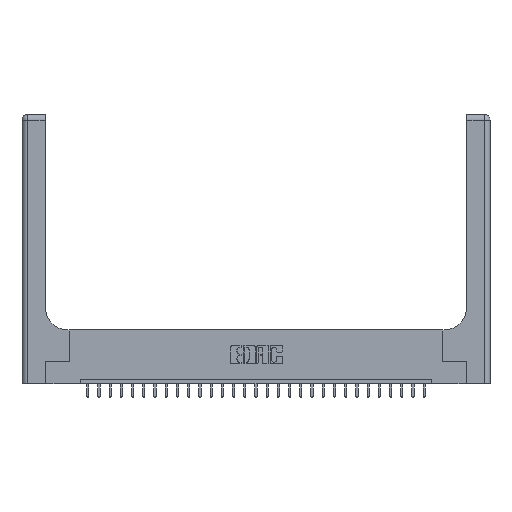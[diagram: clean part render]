
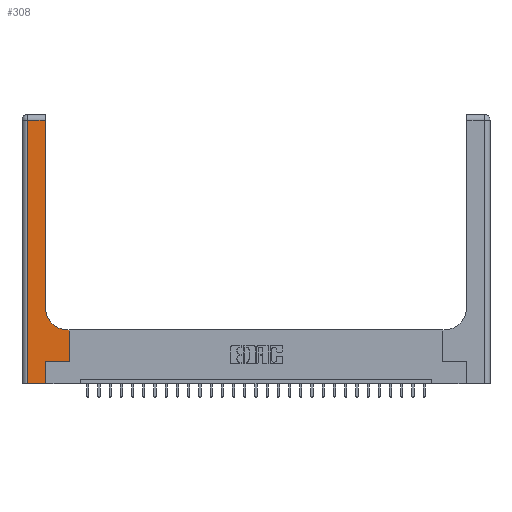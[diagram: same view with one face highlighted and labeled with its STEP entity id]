
A CAD part, top view. The second image highlights one B-rep face of the part: STEP entity #308.
In plain terms, the highlighted planar face has unit normal (0, 0, 1).
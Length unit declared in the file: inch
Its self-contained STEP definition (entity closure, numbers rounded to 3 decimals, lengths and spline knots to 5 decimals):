
#308 = ADVANCED_FACE ( 'NONE', ( #25805 ), #19382, .F. ) ;
#476 = AXIS2_PLACEMENT_3D ( 'NONE', #25495, #11494, #21479 ) ;
#807 = CARTESIAN_POINT ( 'NONE',  ( 0.26, 2.94, 0.37 ) ) ;
#1429 = EDGE_CURVE ( 'NONE', #10382, #23302, #22549, .T. ) ;
#1506 = EDGE_LOOP ( 'NONE', ( #4015, #25766, #17040, #3214, #15412, #5673, #3122, #5263, #17980 ) ) ;
#1592 = VERTEX_POINT ( 'NONE', #12951 ) ;
#2658 = CARTESIAN_POINT ( 'NONE',  ( 0.51, 0.85, 0.37 ) ) ;
#2909 = VECTOR ( 'NONE', #16602, 39.37008 ) ;
#3122 = ORIENTED_EDGE ( 'NONE', *, *, #21930, .T. ) ;
#3214 = ORIENTED_EDGE ( 'NONE', *, *, #24684, .T. ) ;
#3819 = VECTOR ( 'NONE', #23359, 39.37008 ) ;
#3946 = VERTEX_POINT ( 'NONE', #9757 ) ;
#4015 = ORIENTED_EDGE ( 'NONE', *, *, #12102, .T. ) ;
#4040 = CARTESIAN_POINT ( 'NONE',  ( 0.06, 2.94, 0.37 ) ) ;
#4231 = CARTESIAN_POINT ( 'NONE',  ( 0.06, 3., 0.37 ) ) ;
#4755 = CARTESIAN_POINT ( 'NONE',  ( 0.265, 0.25, 0.37 ) ) ;
#5224 = LINE ( 'NONE', #10965, #16913 ) ;
#5263 = ORIENTED_EDGE ( 'NONE', *, *, #16327, .T. ) ;
#5461 = CARTESIAN_POINT ( 'NONE',  ( 0.26, 0.85, 0.37 ) ) ;
#5673 = ORIENTED_EDGE ( 'NONE', *, *, #1429, .T. ) ;
#6763 = CARTESIAN_POINT ( 'NONE',  ( 0.06, 0., 0.37 ) ) ;
#8333 = AXIS2_PLACEMENT_3D ( 'NONE', #2658, #8443, #16576 ) ;
#8377 = LINE ( 'NONE', #18125, #14076 ) ;
#8443 = DIRECTION ( 'NONE',  ( 0., 0., -1. ) ) ;
#9757 = CARTESIAN_POINT ( 'NONE',  ( 0.528, 0.6, 0.37 ) ) ;
#9842 = EDGE_CURVE ( 'NONE', #1592, #21250, #22791, .T. ) ;
#9850 = DIRECTION ( 'NONE',  ( 0., 1., 0. ) ) ;
#9878 = CARTESIAN_POINT ( 'NONE',  ( 0., 2.94, 0.37 ) ) ;
#10382 = VERTEX_POINT ( 'NONE', #21313 ) ;
#10936 = VERTEX_POINT ( 'NONE', #6763 ) ;
#10965 = CARTESIAN_POINT ( 'NONE',  ( 0.265, 0., 0.37 ) ) ;
#11494 = DIRECTION ( 'NONE',  ( 0., 0., -1. ) ) ;
#11501 = VECTOR ( 'NONE', #22801, 39.37008 ) ;
#11527 = EDGE_CURVE ( 'NONE', #16818, #12483, #19607, .T. ) ;
#12102 = EDGE_CURVE ( 'NONE', #21250, #16818, #19269, .T. ) ;
#12483 = VERTEX_POINT ( 'NONE', #4040 ) ;
#12951 = CARTESIAN_POINT ( 'NONE',  ( 0.51, 0.6, 0.37 ) ) ;
#13293 = VECTOR ( 'NONE', #23823, 39.37008 ) ;
#13425 = VERTEX_POINT ( 'NONE', #24651 ) ;
#13594 = LINE ( 'NONE', #24987, #3819 ) ;
#14076 = VECTOR ( 'NONE', #14146, 39.37008 ) ;
#14146 = DIRECTION ( 'NONE',  ( 1., 0., 0. ) ) ;
#15412 = ORIENTED_EDGE ( 'NONE', *, *, #16386, .T. ) ;
#16327 = EDGE_CURVE ( 'NONE', #3946, #1592, #19717, .T. ) ;
#16386 = EDGE_CURVE ( 'NONE', #13425, #10382, #5224, .T. ) ;
#16576 = DIRECTION ( 'NONE',  ( 1., 0., 0. ) ) ;
#16602 = DIRECTION ( 'NONE',  ( 0., -1., 0. ) ) ;
#16804 = CARTESIAN_POINT ( 'NONE',  ( 0.26, 0.6, 0.37 ) ) ;
#16818 = VERTEX_POINT ( 'NONE', #807 ) ;
#16913 = VECTOR ( 'NONE', #17412, 39.37008 ) ;
#17040 = ORIENTED_EDGE ( 'NONE', *, *, #21711, .T. ) ;
#17412 = DIRECTION ( 'NONE',  ( 0., 1., 0. ) ) ;
#17696 = VECTOR ( 'NONE', #9850, 39.37008 ) ;
#17980 = ORIENTED_EDGE ( 'NONE', *, *, #9842, .T. ) ;
#18125 = CARTESIAN_POINT ( 'NONE',  ( 0., 0., 0.37 ) ) ;
#19269 = LINE ( 'NONE', #22421, #17696 ) ;
#19382 = PLANE ( 'NONE',  #476 ) ;
#19607 = LINE ( 'NONE', #9878, #13293 ) ;
#19717 = LINE ( 'NONE', #16804, #11501 ) ;
#21090 = CARTESIAN_POINT ( 'NONE',  ( 0.528, 0.25, 0.37 ) ) ;
#21250 = VERTEX_POINT ( 'NONE', #5461 ) ;
#21313 = CARTESIAN_POINT ( 'NONE',  ( 0.265, 0.25, 0.37 ) ) ;
#21479 = DIRECTION ( 'NONE',  ( -1., 0., 0. ) ) ;
#21711 = EDGE_CURVE ( 'NONE', #12483, #10936, #24237, .T. ) ;
#21930 = EDGE_CURVE ( 'NONE', #23302, #3946, #13594, .T. ) ;
#22421 = CARTESIAN_POINT ( 'NONE',  ( 0.26, 3., 0.37 ) ) ;
#22549 = LINE ( 'NONE', #4755, #24080 ) ;
#22791 = CIRCLE ( 'NONE', #8333, 0.25 ) ;
#22801 = DIRECTION ( 'NONE',  ( -1., 0., 0. ) ) ;
#22950 = DIRECTION ( 'NONE',  ( 1., 0., 0. ) ) ;
#23302 = VERTEX_POINT ( 'NONE', #21090 ) ;
#23359 = DIRECTION ( 'NONE',  ( 0., 1., 0. ) ) ;
#23823 = DIRECTION ( 'NONE',  ( -1., 0., 0. ) ) ;
#24080 = VECTOR ( 'NONE', #22950, 39.37008 ) ;
#24237 = LINE ( 'NONE', #4231, #2909 ) ;
#24651 = CARTESIAN_POINT ( 'NONE',  ( 0.265, 0., 0.37 ) ) ;
#24684 = EDGE_CURVE ( 'NONE', #10936, #13425, #8377, .T. ) ;
#24987 = CARTESIAN_POINT ( 'NONE',  ( 0.528, 0.25, 0.37 ) ) ;
#25495 = CARTESIAN_POINT ( 'NONE',  ( 0., 3., 0.37 ) ) ;
#25766 = ORIENTED_EDGE ( 'NONE', *, *, #11527, .T. ) ;
#25805 = FACE_OUTER_BOUND ( 'NONE', #1506, .T. ) ;
